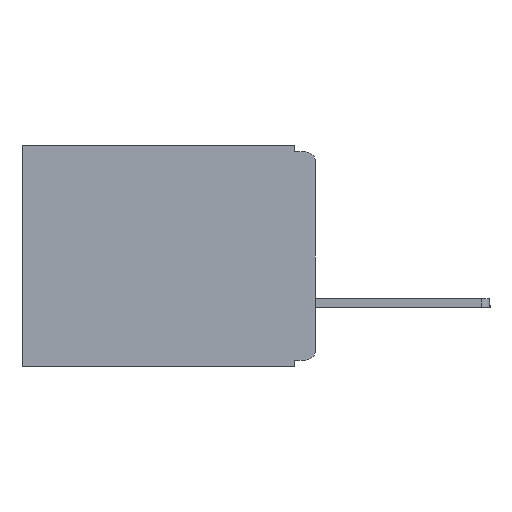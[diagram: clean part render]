
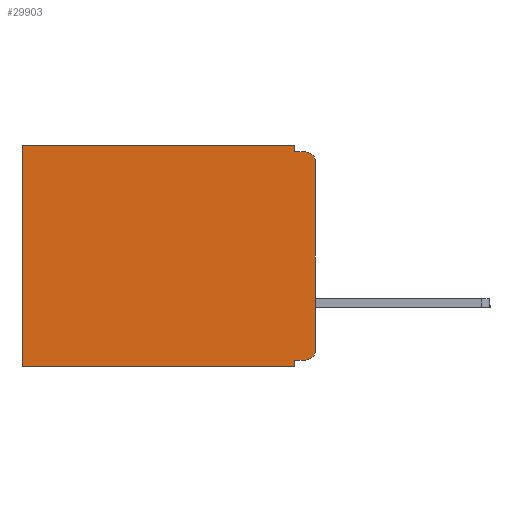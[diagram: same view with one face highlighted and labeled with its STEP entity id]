
A CAD part, left-side view. The second image highlights one B-rep face of the part: STEP entity #29903.
In plain terms, the highlighted planar face has unit normal (-1, 0, 0).
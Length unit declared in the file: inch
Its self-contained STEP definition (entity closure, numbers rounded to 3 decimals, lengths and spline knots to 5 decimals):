
#357 = CARTESIAN_POINT ( 'NONE',  ( 0.3, 0., -0.025 ) ) ;
#761 = CARTESIAN_POINT ( 'NONE',  ( 0.3, 0., -0.33 ) ) ;
#1647 = DIRECTION ( 'NONE',  ( 1., 0., 0. ) ) ;
#2530 = LINE ( 'NONE', #24816, #28464 ) ;
#2763 = ORIENTED_EDGE ( 'NONE', *, *, #13140, .T. ) ;
#3234 = VECTOR ( 'NONE', #10793, 39.37008 ) ;
#3288 = FACE_OUTER_BOUND ( 'NONE', #10898, .T. ) ;
#3598 = VERTEX_POINT ( 'NONE', #25487 ) ;
#3832 = VECTOR ( 'NONE', #23399, 39.37008 ) ;
#4366 = VECTOR ( 'NONE', #9005, 39.37008 ) ;
#4435 = EDGE_CURVE ( 'NONE', #28701, #3598, #19667, .T. ) ;
#4678 = DIRECTION ( 'NONE',  ( 0., 1., 0. ) ) ;
#5389 = CARTESIAN_POINT ( 'NONE',  ( 0.3, 0., 0. ) ) ;
#5612 = EDGE_CURVE ( 'NONE', #28701, #24327, #30142, .T. ) ;
#6154 = VECTOR ( 'NONE', #28012, 39.37008 ) ;
#6317 = ORIENTED_EDGE ( 'NONE', *, *, #5612, .F. ) ;
#6485 = CIRCLE ( 'NONE', #25407, 0.015 ) ;
#6814 = CARTESIAN_POINT ( 'NONE',  ( 0.3, 0.015, -0.025 ) ) ;
#7144 = DIRECTION ( 'NONE',  ( -1., 0., 0. ) ) ;
#7279 = CIRCLE ( 'NONE', #17630, 0.015 ) ;
#7346 = EDGE_CURVE ( 'NONE', #3598, #10698, #2530, .T. ) ;
#7347 = CARTESIAN_POINT ( 'NONE',  ( 0.3, 0.015, -0.32 ) ) ;
#8073 = VERTEX_POINT ( 'NONE', #25544 ) ;
#8100 = VERTEX_POINT ( 'NONE', #25754 ) ;
#8199 = CARTESIAN_POINT ( 'NONE',  ( 0.3, 0., -0.33 ) ) ;
#9005 = DIRECTION ( 'NONE',  ( 0., 0., -1. ) ) ;
#9150 = CARTESIAN_POINT ( 'NONE',  ( 0.3, 0., -0.33 ) ) ;
#9262 = ORIENTED_EDGE ( 'NONE', *, *, #7346, .T. ) ;
#9297 = DIRECTION ( 'NONE',  ( 0., 0., -1. ) ) ;
#9915 = LINE ( 'NONE', #8199, #3234 ) ;
#10698 = VERTEX_POINT ( 'NONE', #26974 ) ;
#10793 = DIRECTION ( 'NONE',  ( 0., 0., -1. ) ) ;
#10898 = EDGE_LOOP ( 'NONE', ( #25352, #2763, #21597, #6317, #30716, #9262, #11529, #11312, #11871, #26677 ) ) ;
#11012 = LINE ( 'NONE', #26558, #4366 ) ;
#11312 = ORIENTED_EDGE ( 'NONE', *, *, #20942, .F. ) ;
#11529 = ORIENTED_EDGE ( 'NONE', *, *, #22893, .F. ) ;
#11871 = ORIENTED_EDGE ( 'NONE', *, *, #18631, .F. ) ;
#12411 = LINE ( 'NONE', #27140, #24968 ) ;
#12716 = EDGE_CURVE ( 'NONE', #19845, #8073, #7279, .T. ) ;
#12800 = LINE ( 'NONE', #20584, #6154 ) ;
#13140 = EDGE_CURVE ( 'NONE', #14733, #14463, #6485, .T. ) ;
#14196 = PLANE ( 'NONE',  #23041 ) ;
#14463 = VERTEX_POINT ( 'NONE', #24242 ) ;
#14572 = VERTEX_POINT ( 'NONE', #27207 ) ;
#14733 = VERTEX_POINT ( 'NONE', #357 ) ;
#17630 = AXIS2_PLACEMENT_3D ( 'NONE', #22148, #7144, #24674 ) ;
#18631 = EDGE_CURVE ( 'NONE', #19845, #8100, #12411, .T. ) ;
#18881 = EDGE_CURVE ( 'NONE', #24327, #14463, #12800, .T. ) ;
#19266 = DIRECTION ( 'NONE',  ( 0., 0., -1. ) ) ;
#19667 = LINE ( 'NONE', #5389, #32099 ) ;
#19845 = VERTEX_POINT ( 'NONE', #7347 ) ;
#19900 = CARTESIAN_POINT ( 'NONE',  ( 0.3, 0.031, -0.01 ) ) ;
#20584 = CARTESIAN_POINT ( 'NONE',  ( 0.3, 0., -0.01 ) ) ;
#20942 = EDGE_CURVE ( 'NONE', #8100, #14572, #11012, .T. ) ;
#21597 = ORIENTED_EDGE ( 'NONE', *, *, #18881, .F. ) ;
#22148 = CARTESIAN_POINT ( 'NONE',  ( 0.3, 0.015, -0.305 ) ) ;
#22893 = EDGE_CURVE ( 'NONE', #14572, #10698, #23832, .T. ) ;
#23041 = AXIS2_PLACEMENT_3D ( 'NONE', #9150, #1647, #19266 ) ;
#23185 = CARTESIAN_POINT ( 'NONE',  ( 0.3, 0.031, 0. ) ) ;
#23332 = CARTESIAN_POINT ( 'NONE',  ( 0.3, 0.031, 0. ) ) ;
#23399 = DIRECTION ( 'NONE',  ( 0., 1., 0. ) ) ;
#23832 = LINE ( 'NONE', #761, #3832 ) ;
#24052 = DIRECTION ( 'NONE',  ( 0., 0., -1. ) ) ;
#24242 = CARTESIAN_POINT ( 'NONE',  ( 0.3, 0.015, -0.01 ) ) ;
#24326 = DIRECTION ( 'NONE',  ( -1., 0., 0. ) ) ;
#24327 = VERTEX_POINT ( 'NONE', #19900 ) ;
#24674 = DIRECTION ( 'NONE',  ( 0., 0., -1. ) ) ;
#24816 = CARTESIAN_POINT ( 'NONE',  ( 0.3, 0.437, -0.33 ) ) ;
#24968 = VECTOR ( 'NONE', #4678, 39.37008 ) ;
#25352 = ORIENTED_EDGE ( 'NONE', *, *, #31439, .F. ) ;
#25407 = AXIS2_PLACEMENT_3D ( 'NONE', #6814, #24326, #9297 ) ;
#25487 = CARTESIAN_POINT ( 'NONE',  ( 0.3, 0.437, 0. ) ) ;
#25544 = CARTESIAN_POINT ( 'NONE',  ( 0.3, 0., -0.305 ) ) ;
#25754 = CARTESIAN_POINT ( 'NONE',  ( 0.3, 0.031, -0.32 ) ) ;
#26558 = CARTESIAN_POINT ( 'NONE',  ( 0.3, 0.031, -0.33 ) ) ;
#26677 = ORIENTED_EDGE ( 'NONE', *, *, #12716, .T. ) ;
#26974 = CARTESIAN_POINT ( 'NONE',  ( 0.3, 0.437, -0.33 ) ) ;
#27140 = CARTESIAN_POINT ( 'NONE',  ( 0.3, 0., -0.32 ) ) ;
#27207 = CARTESIAN_POINT ( 'NONE',  ( 0.3, 0.031, -0.33 ) ) ;
#28012 = DIRECTION ( 'NONE',  ( 0., -1., 0. ) ) ;
#28464 = VECTOR ( 'NONE', #32285, 39.37008 ) ;
#28701 = VERTEX_POINT ( 'NONE', #23332 ) ;
#29363 = VECTOR ( 'NONE', #24052, 39.37008 ) ;
#29903 = ADVANCED_FACE ( 'NONE', ( #3288 ), #14196, .F. ) ;
#30142 = LINE ( 'NONE', #23185, #29363 ) ;
#30151 = DIRECTION ( 'NONE',  ( 0., 1., 0. ) ) ;
#30716 = ORIENTED_EDGE ( 'NONE', *, *, #4435, .T. ) ;
#31439 = EDGE_CURVE ( 'NONE', #14733, #8073, #9915, .T. ) ;
#32099 = VECTOR ( 'NONE', #30151, 39.37008 ) ;
#32285 = DIRECTION ( 'NONE',  ( 0., 0., -1. ) ) ;
